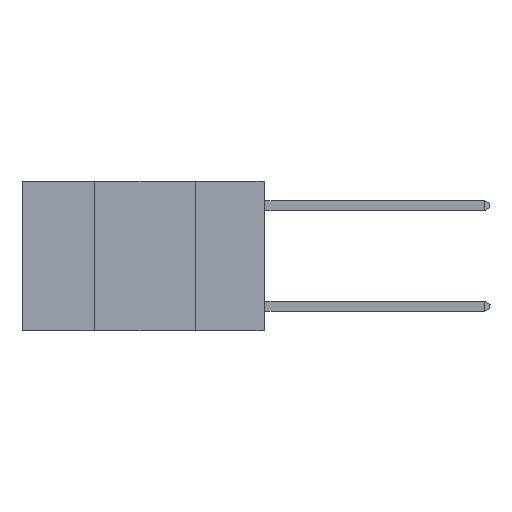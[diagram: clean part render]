
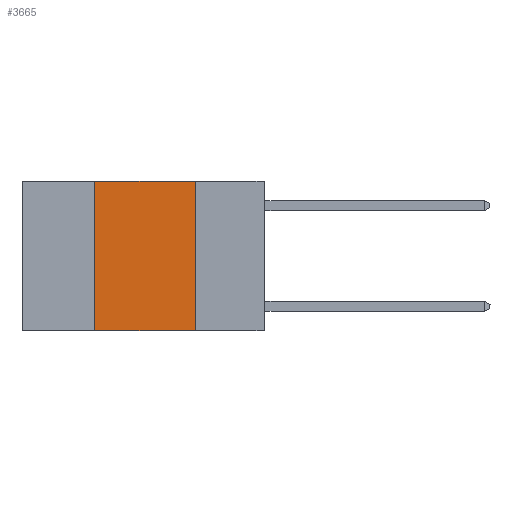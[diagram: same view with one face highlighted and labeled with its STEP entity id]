
A CAD part, left-side view. The second image highlights one B-rep face of the part: STEP entity #3665.
In plain terms, the highlighted planar face has unit normal (-1, 0, 0).
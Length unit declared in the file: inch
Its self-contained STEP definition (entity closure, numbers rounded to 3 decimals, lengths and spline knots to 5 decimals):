
#597 = EDGE_LOOP ( 'NONE', ( #3276, #5505, #7616, #1282 ) ) ;
#765 = VECTOR ( 'NONE', #9174, 39.37008 ) ;
#1282 = ORIENTED_EDGE ( 'NONE', *, *, #3441, .T. ) ;
#1710 = FACE_OUTER_BOUND ( 'NONE', #597, .T. ) ;
#1861 = AXIS2_PLACEMENT_3D ( 'NONE', #10064, #10061, #10052 ) ;
#1942 = CARTESIAN_POINT ( 'NONE',  ( 0., 0.17, 0. ) ) ;
#2044 = VERTEX_POINT ( 'NONE', #1942 ) ;
#2241 = CARTESIAN_POINT ( 'NONE',  ( 0., 0.42, 0. ) ) ;
#2557 = LINE ( 'NONE', #5849, #6756 ) ;
#3276 = ORIENTED_EDGE ( 'NONE', *, *, #3294, .F. ) ;
#3294 = EDGE_CURVE ( 'NONE', #2044, #9175, #7104, .T. ) ;
#3440 = EDGE_CURVE ( 'NONE', #7478, #8019, #10059, .T. ) ;
#3441 = EDGE_CURVE ( 'NONE', #7478, #9175, #5964, .T. ) ;
#3665 = ADVANCED_FACE ( 'NONE', ( #1710 ), #10083, .F. ) ;
#4126 = DIRECTION ( 'NONE',  ( 0., -1., 0. ) ) ;
#4167 = CARTESIAN_POINT ( 'NONE',  ( 0., 0.6, -0.37 ) ) ;
#4391 = DIRECTION ( 'NONE',  ( 0., 0., 1. ) ) ;
#4402 = CARTESIAN_POINT ( 'NONE',  ( 0., 0.42, 0. ) ) ;
#5059 = DIRECTION ( 'NONE',  ( 0., -1., 0. ) ) ;
#5505 = ORIENTED_EDGE ( 'NONE', *, *, #8224, .F. ) ;
#5842 = CARTESIAN_POINT ( 'NONE',  ( 0., 0.17, -0.37 ) ) ;
#5849 = CARTESIAN_POINT ( 'NONE',  ( 0., 0.6, 0. ) ) ;
#5964 = LINE ( 'NONE', #4167, #9828 ) ;
#6600 = CARTESIAN_POINT ( 'NONE',  ( 0., 0.42, -0.37 ) ) ;
#6756 = VECTOR ( 'NONE', #5059, 39.37008 ) ;
#7104 = LINE ( 'NONE', #9092, #765 ) ;
#7478 = VERTEX_POINT ( 'NONE', #6600 ) ;
#7616 = ORIENTED_EDGE ( 'NONE', *, *, #3440, .F. ) ;
#8019 = VERTEX_POINT ( 'NONE', #2241 ) ;
#8224 = EDGE_CURVE ( 'NONE', #8019, #2044, #2557, .T. ) ;
#8303 = VECTOR ( 'NONE', #4391, 39.37008 ) ;
#9092 = CARTESIAN_POINT ( 'NONE',  ( 0., 0.17, 0. ) ) ;
#9174 = DIRECTION ( 'NONE',  ( 0., 0., -1. ) ) ;
#9175 = VERTEX_POINT ( 'NONE', #5842 ) ;
#9828 = VECTOR ( 'NONE', #4126, 39.37008 ) ;
#10052 = DIRECTION ( 'NONE',  ( 0., 0., -1. ) ) ;
#10059 = LINE ( 'NONE', #4402, #8303 ) ;
#10061 = DIRECTION ( 'NONE',  ( 1., 0., 0. ) ) ;
#10064 = CARTESIAN_POINT ( 'NONE',  ( 0., 0.6, 0. ) ) ;
#10083 = PLANE ( 'NONE',  #1861 ) ;
